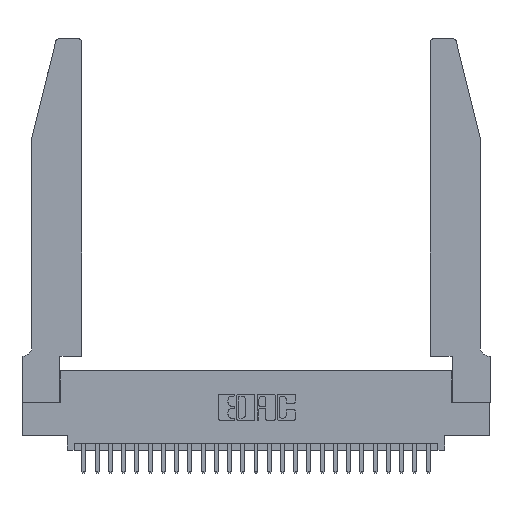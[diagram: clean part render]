
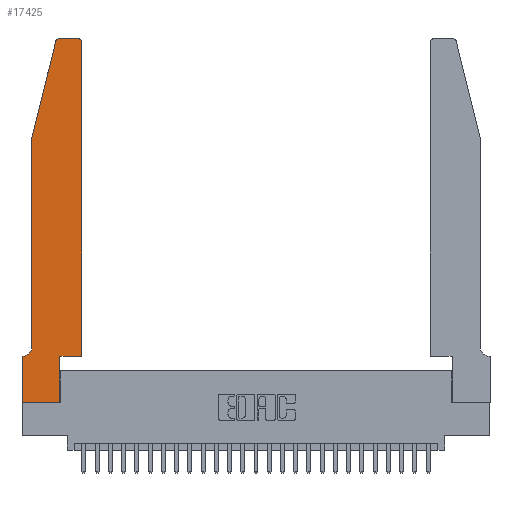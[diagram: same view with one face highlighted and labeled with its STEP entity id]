
A CAD part, top view. The second image highlights one B-rep face of the part: STEP entity #17425.
In plain terms, the highlighted planar face has unit normal (0, 0, 1).
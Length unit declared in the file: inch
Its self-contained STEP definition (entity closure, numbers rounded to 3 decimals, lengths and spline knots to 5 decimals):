
#66 = ORIENTED_EDGE ( 'NONE', *, *, #19516, .T. ) ;
#310 = ORIENTED_EDGE ( 'NONE', *, *, #27834, .T. ) ;
#479 = LINE ( 'NONE', #15034, #23036 ) ;
#676 = EDGE_CURVE ( 'NONE', #3176, #18049, #24028, .T. ) ;
#1511 = AXIS2_PLACEMENT_3D ( 'NONE', #9564, #20639, #24718 ) ;
#1702 = VECTOR ( 'NONE', #7000, 39.37008 ) ;
#1783 = CIRCLE ( 'NONE', #17043, 0.03 ) ;
#2117 = CARTESIAN_POINT ( 'NONE',  ( 0., 0., 0.37 ) ) ;
#2466 = VECTOR ( 'NONE', #15671, 39.37008 ) ;
#2535 = DIRECTION ( 'NONE',  ( 0., 0., 1. ) ) ;
#2544 = CIRCLE ( 'NONE', #21040, 0.07 ) ;
#2813 = DIRECTION ( 'NONE',  ( 1., 0., 0. ) ) ;
#2840 = CARTESIAN_POINT ( 'NONE',  ( 0., 0., 0.37 ) ) ;
#2897 = VECTOR ( 'NONE', #27185, 39.37008 ) ;
#3176 = VERTEX_POINT ( 'NONE', #13803 ) ;
#4711 = VERTEX_POINT ( 'NONE', #24245 ) ;
#4741 = DIRECTION ( 'NONE',  ( -1., 0., 0. ) ) ;
#5307 = DIRECTION ( 'NONE',  ( 0., -1., 0. ) ) ;
#5685 = ORIENTED_EDGE ( 'NONE', *, *, #21433, .T. ) ;
#5713 = CARTESIAN_POINT ( 'NONE',  ( 0.4505, 0.35, 0.37 ) ) ;
#5957 = LINE ( 'NONE', #18527, #2897 ) ;
#6494 = CARTESIAN_POINT ( 'NONE',  ( 0., 0.35, 0.37 ) ) ;
#7000 = DIRECTION ( 'NONE',  ( 1., 0., 0. ) ) ;
#7276 = CARTESIAN_POINT ( 'NONE',  ( 0.4205, 2.72, 0.37 ) ) ;
#8240 = PLANE ( 'NONE',  #17740 ) ;
#8351 = VERTEX_POINT ( 'NONE', #25408 ) ;
#9390 = CARTESIAN_POINT ( 'NONE',  ( 0.25487, 2.72718, 0.37 ) ) ;
#9564 = CARTESIAN_POINT ( 'NONE',  ( 0.284, 2.72, 0.37 ) ) ;
#10215 = ORIENTED_EDGE ( 'NONE', *, *, #12646, .T. ) ;
#10588 = LINE ( 'NONE', #26809, #1702 ) ;
#10596 = DIRECTION ( 'NONE',  ( 1., 0., 0. ) ) ;
#11069 = CARTESIAN_POINT ( 'NONE',  ( 0.0055, 0.42, 0.37 ) ) ;
#11384 = CARTESIAN_POINT ( 'NONE',  ( 0.4505, 0.35, 0.37 ) ) ;
#11925 = CARTESIAN_POINT ( 'NONE',  ( 0.2865, 0.35, 0.37 ) ) ;
#12117 = DIRECTION ( 'NONE',  ( 0., 1., 0. ) ) ;
#12352 = VERTEX_POINT ( 'NONE', #15574 ) ;
#12393 = EDGE_CURVE ( 'NONE', #18049, #14973, #14554, .T. ) ;
#12430 = EDGE_LOOP ( 'NONE', ( #24489, #5685, #22917, #13544, #25345, #20811, #25108, #10215, #26642, #15390, #310, #66 ) ) ;
#12646 = EDGE_CURVE ( 'NONE', #14973, #26715, #26089, .T. ) ;
#12721 = DIRECTION ( 'NONE',  ( 0., 0., 1. ) ) ;
#13098 = VERTEX_POINT ( 'NONE', #23529 ) ;
#13544 = ORIENTED_EDGE ( 'NONE', *, *, #25785, .T. ) ;
#13803 = CARTESIAN_POINT ( 'NONE',  ( 0.0055, 0.35, 0.37 ) ) ;
#14554 = LINE ( 'NONE', #2840, #27466 ) ;
#14901 = DIRECTION ( 'NONE',  ( 0., 1., 0. ) ) ;
#14973 = VERTEX_POINT ( 'NONE', #2117 ) ;
#15034 = CARTESIAN_POINT ( 'NONE',  ( 0.2605, 2.75, 0.37 ) ) ;
#15334 = EDGE_CURVE ( 'NONE', #25300, #12352, #16477, .T. ) ;
#15390 = ORIENTED_EDGE ( 'NONE', *, *, #21289, .T. ) ;
#15574 = CARTESIAN_POINT ( 'NONE',  ( 0.0755, 2., 0.37 ) ) ;
#15671 = DIRECTION ( 'NONE',  ( -0.239, -0.971, 0. ) ) ;
#15738 = CIRCLE ( 'NONE', #1511, 0.03 ) ;
#16477 = LINE ( 'NONE', #26218, #2466 ) ;
#17043 = AXIS2_PLACEMENT_3D ( 'NONE', #7276, #2535, #2813 ) ;
#17067 = CARTESIAN_POINT ( 'NONE',  ( 0.2865, 0., 0.37 ) ) ;
#17425 = ADVANCED_FACE ( 'NONE', ( #27551 ), #8240, .T. ) ;
#17710 = CARTESIAN_POINT ( 'NONE',  ( 0.284, 2.75, 0.37 ) ) ;
#17740 = AXIS2_PLACEMENT_3D ( 'NONE', #25962, #12721, #21384 ) ;
#18049 = VERTEX_POINT ( 'NONE', #6494 ) ;
#18168 = EDGE_CURVE ( 'NONE', #23214, #3176, #2544, .T. ) ;
#18217 = VECTOR ( 'NONE', #20612, 39.37008 ) ;
#18527 = CARTESIAN_POINT ( 'NONE',  ( 0.0755, 2., 0.37 ) ) ;
#18787 = VECTOR ( 'NONE', #12117, 39.37008 ) ;
#19516 = EDGE_CURVE ( 'NONE', #8351, #13098, #1783, .T. ) ;
#20300 = VECTOR ( 'NONE', #10596, 39.37008 ) ;
#20412 = CARTESIAN_POINT ( 'NONE',  ( 0.0755, 0.35, 0.37 ) ) ;
#20420 = EDGE_CURVE ( 'NONE', #26715, #4711, #20851, .T. ) ;
#20612 = DIRECTION ( 'NONE',  ( -1., 0., 0. ) ) ;
#20639 = DIRECTION ( 'NONE',  ( 0., 0., 1. ) ) ;
#20811 = ORIENTED_EDGE ( 'NONE', *, *, #676, .T. ) ;
#20851 = LINE ( 'NONE', #11925, #18787 ) ;
#21040 = AXIS2_PLACEMENT_3D ( 'NONE', #11069, #21924, #4741 ) ;
#21289 = EDGE_CURVE ( 'NONE', #4711, #24225, #10588, .T. ) ;
#21361 = CARTESIAN_POINT ( 'NONE',  ( 0., 0., 0.37 ) ) ;
#21384 = DIRECTION ( 'NONE',  ( 1., 0., 0. ) ) ;
#21433 = EDGE_CURVE ( 'NONE', #25158, #25300, #15738, .T. ) ;
#21924 = DIRECTION ( 'NONE',  ( 0., 0., -1. ) ) ;
#22791 = CARTESIAN_POINT ( 'NONE',  ( 0.0755, 0.42, 0.37 ) ) ;
#22917 = ORIENTED_EDGE ( 'NONE', *, *, #15334, .T. ) ;
#23036 = VECTOR ( 'NONE', #23865, 39.37008 ) ;
#23214 = VERTEX_POINT ( 'NONE', #22791 ) ;
#23286 = LINE ( 'NONE', #5713, #26014 ) ;
#23529 = CARTESIAN_POINT ( 'NONE',  ( 0.4205, 2.75, 0.37 ) ) ;
#23865 = DIRECTION ( 'NONE',  ( -1., 0., 0. ) ) ;
#24028 = LINE ( 'NONE', #20412, #18217 ) ;
#24225 = VERTEX_POINT ( 'NONE', #11384 ) ;
#24245 = CARTESIAN_POINT ( 'NONE',  ( 0.2865, 0.35, 0.37 ) ) ;
#24489 = ORIENTED_EDGE ( 'NONE', *, *, #26025, .T. ) ;
#24718 = DIRECTION ( 'NONE',  ( 1., 0., 0. ) ) ;
#25108 = ORIENTED_EDGE ( 'NONE', *, *, #12393, .T. ) ;
#25158 = VERTEX_POINT ( 'NONE', #17710 ) ;
#25300 = VERTEX_POINT ( 'NONE', #9390 ) ;
#25345 = ORIENTED_EDGE ( 'NONE', *, *, #18168, .T. ) ;
#25408 = CARTESIAN_POINT ( 'NONE',  ( 0.4505, 2.72, 0.37 ) ) ;
#25785 = EDGE_CURVE ( 'NONE', #12352, #23214, #5957, .T. ) ;
#25962 = CARTESIAN_POINT ( 'NONE',  ( 0., 0.35, 0.37 ) ) ;
#26014 = VECTOR ( 'NONE', #14901, 39.37008 ) ;
#26025 = EDGE_CURVE ( 'NONE', #13098, #25158, #479, .T. ) ;
#26089 = LINE ( 'NONE', #21361, #20300 ) ;
#26218 = CARTESIAN_POINT ( 'NONE',  ( 0.0755, 2., 0.37 ) ) ;
#26642 = ORIENTED_EDGE ( 'NONE', *, *, #20420, .T. ) ;
#26715 = VERTEX_POINT ( 'NONE', #17067 ) ;
#26809 = CARTESIAN_POINT ( 'NONE',  ( 0.4505, 0.35, 0.37 ) ) ;
#27185 = DIRECTION ( 'NONE',  ( 0., -1., 0. ) ) ;
#27466 = VECTOR ( 'NONE', #5307, 39.37008 ) ;
#27551 = FACE_OUTER_BOUND ( 'NONE', #12430, .T. ) ;
#27834 = EDGE_CURVE ( 'NONE', #24225, #8351, #23286, .T. ) ;
